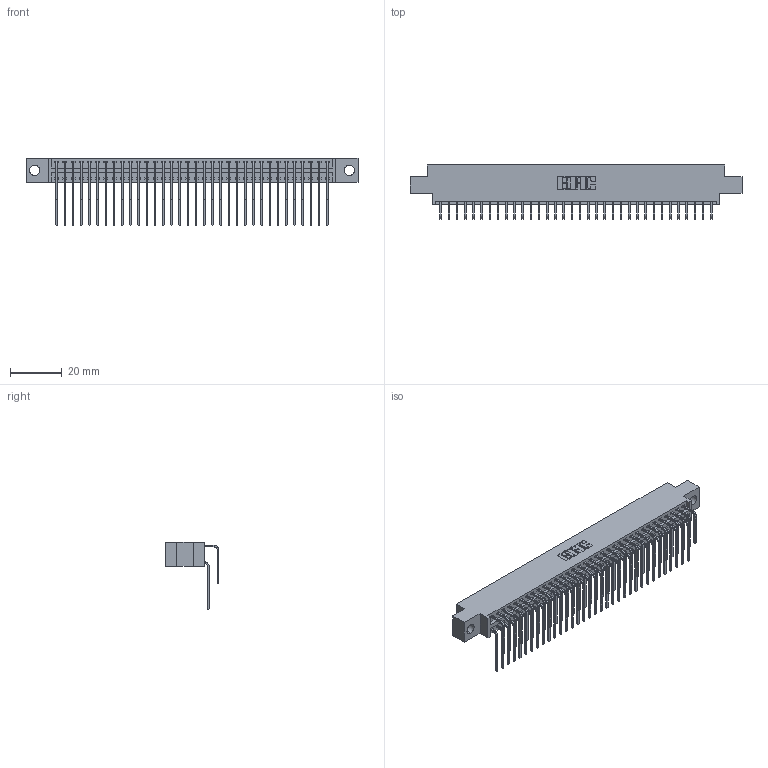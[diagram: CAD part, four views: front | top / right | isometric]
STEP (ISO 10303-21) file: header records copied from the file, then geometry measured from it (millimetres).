
FILE_DESCRIPTION (( 'STEP AP203' ), '1' );
FILE_NAME ('346-068-559-804.STEP', '2018-08-28T22:32:51', ( '' ), ( '' ), 'SwSTEP 2.0', 'SolidWorks 2016', '' );
FILE_SCHEMA (( 'CONFIG_CONTROL_DESIGN' ));
Length unit declared in the file: inch
Products named in the file (4): 346 Part_0.170 Offset - 0.156 Dia-TH; 345-292-001_558 559 Tail - 1; 345-292-001_559 Tail - 2; 346-068-559-804
Assembly tree (69 placements, depth 2):
  346-068-559-804
    346 Part_0.170 Offset - 0.156 Dia-TH
    345-292-001_558 559 Tail - 1  x34
    345-292-001_559 Tail - 2  x34
Bounding box: 128.52 x 20.89 x 26.16 mm (x, y, z)
Volume: 12620.4 mm3; surface area: 19096.6 mm2
Topology: 69 solids, 69 shells, 3798 faces, 11289 edges, 7434 vertices
Faces by surface type: plane 2596, cylinder 1202
Entity records: 25185 total; most frequent: CARTESIAN_POINT 4215, ORIENTED_EDGE 4098, DIRECTION 3737, EDGE_CURVE 2049, LINE 1741, VECTOR 1741, VERTEX_POINT 1362, AXIS2_PLACEMENT_3D 998
